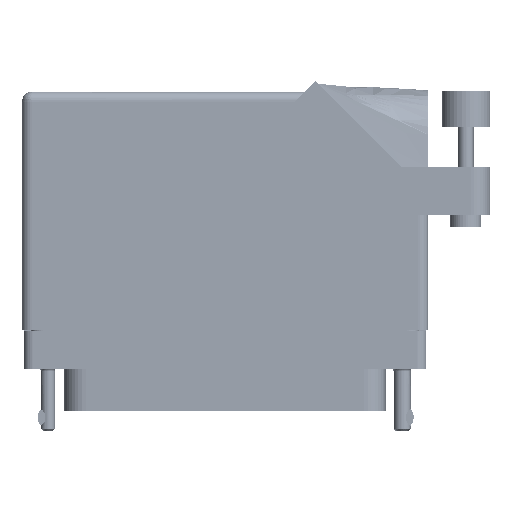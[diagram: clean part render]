
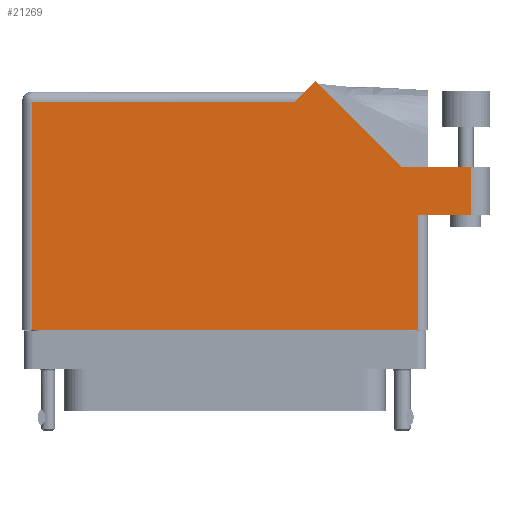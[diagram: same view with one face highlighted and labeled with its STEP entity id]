
A CAD part, front view. The second image highlights one B-rep face of the part: STEP entity #21269.
In plain terms, the highlighted face is planar.
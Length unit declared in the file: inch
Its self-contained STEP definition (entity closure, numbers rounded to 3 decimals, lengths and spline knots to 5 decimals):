
#1564 = CARTESIAN_POINT ( 'NONE',  ( -1.306, 1.43, 0.455 ) ) ;
#1695 = VECTOR ( 'NONE', #17047, 39.37008 ) ;
#1903 = CARTESIAN_POINT ( 'NONE',  ( -1.244, 1.368, 0.455 ) ) ;
#3185 = VECTOR ( 'NONE', #29502, 39.37008 ) ;
#3313 = VERTEX_POINT ( 'NONE', #37248 ) ;
#4182 = LINE ( 'NONE', #15154, #7828 ) ;
#6078 = ORIENTED_EDGE ( 'NONE', *, *, #21739, .T. ) ;
#6774 = CARTESIAN_POINT ( 'NONE',  ( 1.14042, 0.944, 0.455 ) ) ;
#7828 = VECTOR ( 'NONE', #29024, 39.37008 ) ;
#7854 = ORIENTED_EDGE ( 'NONE', *, *, #60412, .T. ) ;
#8149 = CARTESIAN_POINT ( 'NONE',  ( 1.244, -0.1, 0.455 ) ) ;
#8511 = FACE_OUTER_BOUND ( 'NONE', #22699, .T. ) ;
#10364 = CARTESIAN_POINT ( 'NONE',  ( 0.58371, 1.50071, 0.455 ) ) ;
#11572 = LINE ( 'NONE', #44160, #32311 ) ;
#12344 = ORIENTED_EDGE ( 'NONE', *, *, #14579, .T. ) ;
#13160 = DIRECTION ( 'NONE',  ( -1., 0., 0. ) ) ;
#14060 = ORIENTED_EDGE ( 'NONE', *, *, #51071, .T. ) ;
#14579 = EDGE_CURVE ( 'NONE', #23509, #54024, #4182, .T. ) ;
#15154 = CARTESIAN_POINT ( 'NONE',  ( 0.513, 1.43, 0.455 ) ) ;
#15520 = ORIENTED_EDGE ( 'NONE', *, *, #40520, .T. ) ;
#15577 = VERTEX_POINT ( 'NONE', #8149 ) ;
#15680 = DIRECTION ( 'NONE',  ( 0., 0., -1. ) ) ;
#15942 = DIRECTION ( 'NONE',  ( -1., 0., 0. ) ) ;
#16479 = CARTESIAN_POINT ( 'NONE',  ( 1.14042, 0.944, 0.455 ) ) ;
#16609 = LINE ( 'NONE', #26889, #38904 ) ;
#17047 = DIRECTION ( 'NONE',  ( 1., 0., 0. ) ) ;
#19596 = CARTESIAN_POINT ( 'NONE',  ( 1.581, 0.944, 0.455 ) ) ;
#20040 = DIRECTION ( 'NONE',  ( -1., 0., 0. ) ) ;
#21132 = LINE ( 'NONE', #60183, #47831 ) ;
#21269 = ADVANCED_FACE ( 'NONE', ( #8511 ), #23772, .F. ) ;
#21373 = VECTOR ( 'NONE', #43919, 39.37008 ) ;
#21739 = EDGE_CURVE ( 'NONE', #48505, #36776, #16609, .T. ) ;
#22066 = EDGE_CURVE ( 'NONE', #54024, #53264, #59512, .T. ) ;
#22358 = AXIS2_PLACEMENT_3D ( 'NONE', #1564, #15680, #20040 ) ;
#22558 = DIRECTION ( 'NONE',  ( 1., 0., 0. ) ) ;
#22699 = EDGE_LOOP ( 'NONE', ( #6078, #24450, #7854, #15520, #12344, #31315, #38599, #14060, #46703 ) ) ;
#23333 = CARTESIAN_POINT ( 'NONE',  ( 0.451, 1.368, 0.455 ) ) ;
#23509 = VERTEX_POINT ( 'NONE', #10364 ) ;
#23772 = PLANE ( 'NONE',  #22358 ) ;
#24450 = ORIENTED_EDGE ( 'NONE', *, *, #28552, .T. ) ;
#25505 = DIRECTION ( 'NONE',  ( 0., 1., 0. ) ) ;
#26889 = CARTESIAN_POINT ( 'NONE',  ( 1.306, 0.637, 0.455 ) ) ;
#28552 = EDGE_CURVE ( 'NONE', #36776, #3313, #31346, .T. ) ;
#28803 = VECTOR ( 'NONE', #25505, 39.37008 ) ;
#29024 = DIRECTION ( 'NONE',  ( -0.707, -0.707, 0. ) ) ;
#29502 = DIRECTION ( 'NONE',  ( 0., 1., 0. ) ) ;
#30173 = CARTESIAN_POINT ( 'NONE',  ( 1.244, 0.637, 0.455 ) ) ;
#31315 = ORIENTED_EDGE ( 'NONE', *, *, #22066, .T. ) ;
#31346 = LINE ( 'NONE', #19596, #3185 ) ;
#32021 = CARTESIAN_POINT ( 'NONE',  ( -1.306, 1.368, 0.455 ) ) ;
#32143 = DIRECTION ( 'NONE',  ( 0., -1., 0. ) ) ;
#32311 = VECTOR ( 'NONE', #15942, 39.37008 ) ;
#32563 = LINE ( 'NONE', #39618, #28803 ) ;
#36776 = VERTEX_POINT ( 'NONE', #54166 ) ;
#37248 = CARTESIAN_POINT ( 'NONE',  ( 1.581, 0.944, 0.455 ) ) ;
#38599 = ORIENTED_EDGE ( 'NONE', *, *, #61089, .T. ) ;
#38904 = VECTOR ( 'NONE', #22558, 39.37008 ) ;
#39618 = CARTESIAN_POINT ( 'NONE',  ( 1.244, 0.637, 0.455 ) ) ;
#40092 = EDGE_CURVE ( 'NONE', #15577, #48505, #32563, .T. ) ;
#40520 = EDGE_CURVE ( 'NONE', #52560, #23509, #46589, .T. ) ;
#42662 = VECTOR ( 'NONE', #13160, 39.37008 ) ;
#43919 = DIRECTION ( 'NONE',  ( -0.707, 0.707, 0. ) ) ;
#44160 = CARTESIAN_POINT ( 'NONE',  ( 1.706, 0.944, 0.455 ) ) ;
#46589 = LINE ( 'NONE', #6774, #21373 ) ;
#46703 = ORIENTED_EDGE ( 'NONE', *, *, #40092, .T. ) ;
#47831 = VECTOR ( 'NONE', #32143, 39.37008 ) ;
#48505 = VERTEX_POINT ( 'NONE', #30173 ) ;
#49070 = CARTESIAN_POINT ( 'NONE',  ( -1.244, -0.1, 0.455 ) ) ;
#51071 = EDGE_CURVE ( 'NONE', #57025, #15577, #60890, .T. ) ;
#52560 = VERTEX_POINT ( 'NONE', #16479 ) ;
#53264 = VERTEX_POINT ( 'NONE', #1903 ) ;
#54024 = VERTEX_POINT ( 'NONE', #23333 ) ;
#54166 = CARTESIAN_POINT ( 'NONE',  ( 1.581, 0.637, 0.455 ) ) ;
#57025 = VERTEX_POINT ( 'NONE', #49070 ) ;
#59161 = CARTESIAN_POINT ( 'NONE',  ( -1.306, -0.1, 0.455 ) ) ;
#59512 = LINE ( 'NONE', #32021, #42662 ) ;
#60183 = CARTESIAN_POINT ( 'NONE',  ( -1.244, -0.1, 0.455 ) ) ;
#60412 = EDGE_CURVE ( 'NONE', #3313, #52560, #11572, .T. ) ;
#60890 = LINE ( 'NONE', #59161, #1695 ) ;
#61089 = EDGE_CURVE ( 'NONE', #53264, #57025, #21132, .T. ) ;
